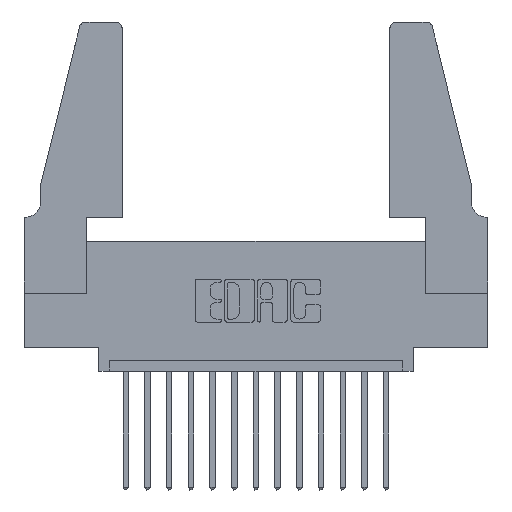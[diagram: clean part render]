
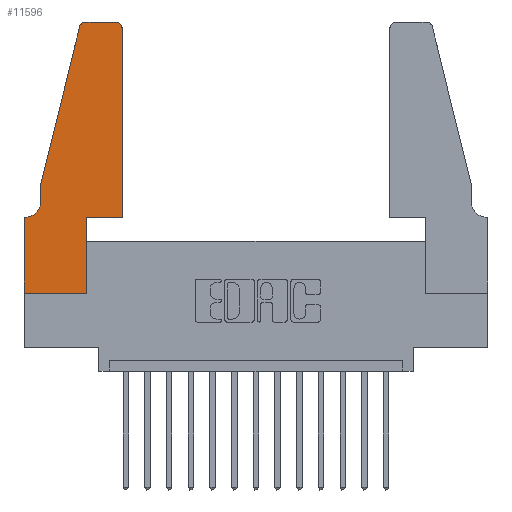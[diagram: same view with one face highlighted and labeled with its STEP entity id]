
A CAD part, top view. The second image highlights one B-rep face of the part: STEP entity #11596.
In plain terms, the highlighted planar face has unit normal (0, 0, 1).
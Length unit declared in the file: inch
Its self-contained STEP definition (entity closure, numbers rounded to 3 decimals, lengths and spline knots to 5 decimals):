
#113 = VERTEX_POINT ( 'NONE', #3317 ) ;
#179 = DIRECTION ( 'NONE',  ( 0., -1., 0. ) ) ;
#448 = VERTEX_POINT ( 'NONE', #13749 ) ;
#515 = VERTEX_POINT ( 'NONE', #7928 ) ;
#580 = CARTESIAN_POINT ( 'NONE',  ( 0.0755, 0.5, 0.37 ) ) ;
#618 = DIRECTION ( 'NONE',  ( 0., 1., 0. ) ) ;
#786 = CARTESIAN_POINT ( 'NONE',  ( 0.2605, 1.25, 0.37 ) ) ;
#789 = CIRCLE ( 'NONE', #11223, 0.03 ) ;
#885 = AXIS2_PLACEMENT_3D ( 'NONE', #5050, #3614, #4959 ) ;
#1093 = CIRCLE ( 'NONE', #885, 0.07 ) ;
#1125 = EDGE_CURVE ( 'NONE', #6826, #448, #13012, .T. ) ;
#1580 = VERTEX_POINT ( 'NONE', #7690 ) ;
#1770 = CARTESIAN_POINT ( 'NONE',  ( 0.284, 1.22, 0.37 ) ) ;
#1880 = CARTESIAN_POINT ( 'NONE',  ( 0., 0., 0.37 ) ) ;
#2073 = VERTEX_POINT ( 'NONE', #9924 ) ;
#2728 = CARTESIAN_POINT ( 'NONE',  ( 0.0755, 0.5, 0.37 ) ) ;
#3038 = VERTEX_POINT ( 'NONE', #3509 ) ;
#3150 = CARTESIAN_POINT ( 'NONE',  ( 0.4505, 0.35, 0.37 ) ) ;
#3260 = ORIENTED_EDGE ( 'NONE', *, *, #14751, .T. ) ;
#3317 = CARTESIAN_POINT ( 'NONE',  ( 0., 0., 0.37 ) ) ;
#3367 = CARTESIAN_POINT ( 'NONE',  ( 0., 0.35, 0.37 ) ) ;
#3509 = CARTESIAN_POINT ( 'NONE',  ( 0.25487, 1.22718, 0.37 ) ) ;
#3614 = DIRECTION ( 'NONE',  ( 0., 0., -1. ) ) ;
#3769 = EDGE_CURVE ( 'NONE', #515, #113, #15477, .T. ) ;
#3785 = VECTOR ( 'NONE', #6268, 39.37008 ) ;
#3808 = VECTOR ( 'NONE', #10394, 39.37008 ) ;
#4051 = EDGE_CURVE ( 'NONE', #448, #1580, #5839, .T. ) ;
#4053 = VERTEX_POINT ( 'NONE', #15764 ) ;
#4079 = DIRECTION ( 'NONE',  ( -0.239, -0.971, 0. ) ) ;
#4161 = CARTESIAN_POINT ( 'NONE',  ( 0., 0., 0.37 ) ) ;
#4450 = VECTOR ( 'NONE', #618, 39.37008 ) ;
#4528 = EDGE_CURVE ( 'NONE', #1580, #2073, #11763, .T. ) ;
#4792 = EDGE_CURVE ( 'NONE', #2073, #7410, #789, .T. ) ;
#4958 = LINE ( 'NONE', #786, #7231 ) ;
#4959 = DIRECTION ( 'NONE',  ( -1., 0., 0. ) ) ;
#5050 = CARTESIAN_POINT ( 'NONE',  ( 0.0055, 0.42, 0.37 ) ) ;
#5144 = LINE ( 'NONE', #580, #3808 ) ;
#5271 = ORIENTED_EDGE ( 'NONE', *, *, #4051, .T. ) ;
#5468 = EDGE_LOOP ( 'NONE', ( #7715, #6898, #5742, #10137, #9006, #3260, #7164, #14607, #12063, #5271, #8532, #15878 ) ) ;
#5742 = ORIENTED_EDGE ( 'NONE', *, *, #12356, .T. ) ;
#5839 = LINE ( 'NONE', #6014, #6582 ) ;
#5968 = DIRECTION ( 'NONE',  ( 0., 0., 1. ) ) ;
#6014 = CARTESIAN_POINT ( 'NONE',  ( 0.4505, 0.35, 0.37 ) ) ;
#6048 = VERTEX_POINT ( 'NONE', #2728 ) ;
#6268 = DIRECTION ( 'NONE',  ( 0., 1., 0. ) ) ;
#6582 = VECTOR ( 'NONE', #13429, 39.37008 ) ;
#6639 = VECTOR ( 'NONE', #13406, 39.37008 ) ;
#6736 = CARTESIAN_POINT ( 'NONE',  ( 0.0755, 0.35, 0.37 ) ) ;
#6756 = CARTESIAN_POINT ( 'NONE',  ( 0.0755, 0.5, 0.37 ) ) ;
#6800 = FACE_OUTER_BOUND ( 'NONE', #5468, .T. ) ;
#6826 = VERTEX_POINT ( 'NONE', #8628 ) ;
#6898 = ORIENTED_EDGE ( 'NONE', *, *, #14945, .T. ) ;
#7062 = CARTESIAN_POINT ( 'NONE',  ( 0.4205, 1.22, 0.37 ) ) ;
#7126 = CARTESIAN_POINT ( 'NONE',  ( 0.0055, 0.35, 0.37 ) ) ;
#7164 = ORIENTED_EDGE ( 'NONE', *, *, #3769, .T. ) ;
#7231 = VECTOR ( 'NONE', #9346, 39.37008 ) ;
#7276 = AXIS2_PLACEMENT_3D ( 'NONE', #3367, #11802, #10747 ) ;
#7372 = VERTEX_POINT ( 'NONE', #7126 ) ;
#7410 = VERTEX_POINT ( 'NONE', #15886 ) ;
#7579 = CARTESIAN_POINT ( 'NONE',  ( 0.0755, 0.42, 0.37 ) ) ;
#7690 = CARTESIAN_POINT ( 'NONE',  ( 0.4505, 0.35, 0.37 ) ) ;
#7715 = ORIENTED_EDGE ( 'NONE', *, *, #14345, .T. ) ;
#7900 = DIRECTION ( 'NONE',  ( 1., 0., 0. ) ) ;
#7928 = CARTESIAN_POINT ( 'NONE',  ( 0., 0.35, 0.37 ) ) ;
#8532 = ORIENTED_EDGE ( 'NONE', *, *, #4528, .T. ) ;
#8628 = CARTESIAN_POINT ( 'NONE',  ( 0.2865, 0., 0.37 ) ) ;
#9006 = ORIENTED_EDGE ( 'NONE', *, *, #9828, .T. ) ;
#9346 = DIRECTION ( 'NONE',  ( -1., 0., 0. ) ) ;
#9499 = DIRECTION ( 'NONE',  ( 1., 0., 0. ) ) ;
#9724 = VECTOR ( 'NONE', #7900, 39.37008 ) ;
#9828 = EDGE_CURVE ( 'NONE', #11897, #7372, #1093, .T. ) ;
#9846 = CARTESIAN_POINT ( 'NONE',  ( 0.2865, 0.35, 0.37 ) ) ;
#9924 = CARTESIAN_POINT ( 'NONE',  ( 0.4505, 1.22, 0.37 ) ) ;
#10137 = ORIENTED_EDGE ( 'NONE', *, *, #13360, .T. ) ;
#10394 = DIRECTION ( 'NONE',  ( 0., -1., 0. ) ) ;
#10747 = DIRECTION ( 'NONE',  ( 1., 0., 0. ) ) ;
#10800 = DIRECTION ( 'NONE',  ( 0., 0., 1. ) ) ;
#10879 = LINE ( 'NONE', #6756, #14017 ) ;
#11177 = VECTOR ( 'NONE', #179, 39.37008 ) ;
#11223 = AXIS2_PLACEMENT_3D ( 'NONE', #7062, #10800, #9499 ) ;
#11455 = CIRCLE ( 'NONE', #14203, 0.03 ) ;
#11596 = ADVANCED_FACE ( 'NONE', ( #6800 ), #15594, .T. ) ;
#11763 = LINE ( 'NONE', #3150, #4450 ) ;
#11802 = DIRECTION ( 'NONE',  ( 0., 0., 1. ) ) ;
#11897 = VERTEX_POINT ( 'NONE', #7579 ) ;
#12063 = ORIENTED_EDGE ( 'NONE', *, *, #1125, .T. ) ;
#12310 = LINE ( 'NONE', #1880, #9724 ) ;
#12356 = EDGE_CURVE ( 'NONE', #3038, #6048, #10879, .T. ) ;
#12421 = EDGE_CURVE ( 'NONE', #113, #6826, #12310, .T. ) ;
#13012 = LINE ( 'NONE', #9846, #3785 ) ;
#13360 = EDGE_CURVE ( 'NONE', #6048, #11897, #5144, .T. ) ;
#13406 = DIRECTION ( 'NONE',  ( -1., 0., 0. ) ) ;
#13429 = DIRECTION ( 'NONE',  ( 1., 0., 0. ) ) ;
#13749 = CARTESIAN_POINT ( 'NONE',  ( 0.2865, 0.35, 0.37 ) ) ;
#14017 = VECTOR ( 'NONE', #4079, 39.37008 ) ;
#14163 = DIRECTION ( 'NONE',  ( 1., 0., 0. ) ) ;
#14203 = AXIS2_PLACEMENT_3D ( 'NONE', #1770, #5968, #14163 ) ;
#14345 = EDGE_CURVE ( 'NONE', #7410, #4053, #4958, .T. ) ;
#14607 = ORIENTED_EDGE ( 'NONE', *, *, #12421, .T. ) ;
#14751 = EDGE_CURVE ( 'NONE', #7372, #515, #15930, .T. ) ;
#14945 = EDGE_CURVE ( 'NONE', #4053, #3038, #11455, .T. ) ;
#15477 = LINE ( 'NONE', #4161, #11177 ) ;
#15594 = PLANE ( 'NONE',  #7276 ) ;
#15764 = CARTESIAN_POINT ( 'NONE',  ( 0.284, 1.25, 0.37 ) ) ;
#15878 = ORIENTED_EDGE ( 'NONE', *, *, #4792, .T. ) ;
#15886 = CARTESIAN_POINT ( 'NONE',  ( 0.4205, 1.25, 0.37 ) ) ;
#15930 = LINE ( 'NONE', #6736, #6639 ) ;
